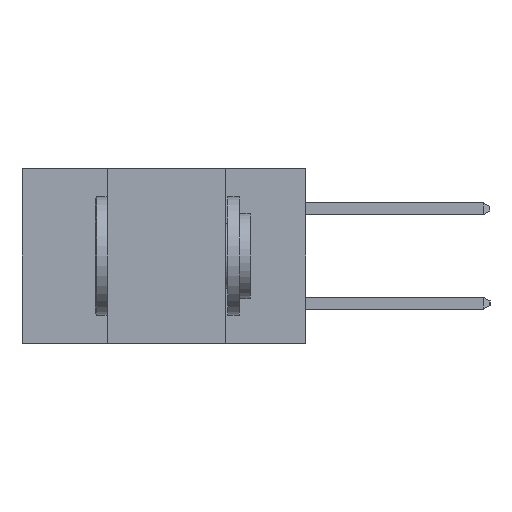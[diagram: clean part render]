
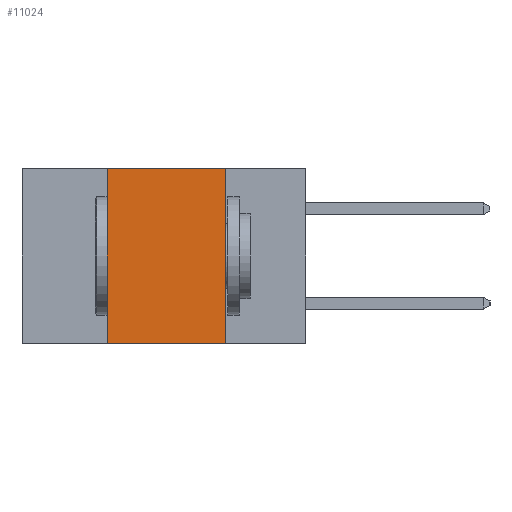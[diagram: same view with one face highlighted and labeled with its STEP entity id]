
A CAD part, left-side view. The second image highlights one B-rep face of the part: STEP entity #11024.
In plain terms, the highlighted planar face has unit normal (-1, 0, 0).
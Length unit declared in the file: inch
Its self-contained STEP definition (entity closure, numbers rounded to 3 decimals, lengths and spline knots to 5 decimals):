
#411 = CARTESIAN_POINT ( 'NONE',  ( 0., 0.6, 0. ) ) ;
#807 = VERTEX_POINT ( 'NONE', #8865 ) ;
#871 = VECTOR ( 'NONE', #3319, 39.37008 ) ;
#1193 = CARTESIAN_POINT ( 'NONE',  ( 0., 0.6, -0.37 ) ) ;
#2861 = VECTOR ( 'NONE', #19560, 39.37008 ) ;
#3172 = ORIENTED_EDGE ( 'NONE', *, *, #22668, .T. ) ;
#3319 = DIRECTION ( 'NONE',  ( 0., -1., 0. ) ) ;
#3367 = CARTESIAN_POINT ( 'NONE',  ( 0., 0.17, -0.37 ) ) ;
#3524 = LINE ( 'NONE', #15432, #2861 ) ;
#3663 = DIRECTION ( 'NONE',  ( 0., 0., -1. ) ) ;
#4638 = DIRECTION ( 'NONE',  ( 0., 0., -1. ) ) ;
#4787 = LINE ( 'NONE', #19013, #24238 ) ;
#7179 = ORIENTED_EDGE ( 'NONE', *, *, #15148, .F. ) ;
#7495 = CARTESIAN_POINT ( 'NONE',  ( 0., 0.42, -0.37 ) ) ;
#7552 = VECTOR ( 'NONE', #3663, 39.37008 ) ;
#8211 = LINE ( 'NONE', #11925, #7552 ) ;
#8865 = CARTESIAN_POINT ( 'NONE',  ( 0., 0.17, 0. ) ) ;
#10046 = AXIS2_PLACEMENT_3D ( 'NONE', #411, #17106, #4638 ) ;
#11024 = ADVANCED_FACE ( 'NONE', ( #21280 ), #15019, .F. ) ;
#11292 = VERTEX_POINT ( 'NONE', #3367 ) ;
#11925 = CARTESIAN_POINT ( 'NONE',  ( 0., 0.17, -0.37 ) ) ;
#12518 = VERTEX_POINT ( 'NONE', #25658 ) ;
#12918 = DIRECTION ( 'NONE',  ( 0., -1., 0. ) ) ;
#13520 = EDGE_LOOP ( 'NONE', ( #7179, #23000, #16839, #3172 ) ) ;
#15019 = PLANE ( 'NONE',  #10046 ) ;
#15148 = EDGE_CURVE ( 'NONE', #807, #11292, #8211, .T. ) ;
#15432 = CARTESIAN_POINT ( 'NONE',  ( 0., 0.42, -0.37 ) ) ;
#16839 = ORIENTED_EDGE ( 'NONE', *, *, #18507, .F. ) ;
#17106 = DIRECTION ( 'NONE',  ( 1., 0., 0. ) ) ;
#17209 = VERTEX_POINT ( 'NONE', #7495 ) ;
#18160 = LINE ( 'NONE', #1193, #871 ) ;
#18507 = EDGE_CURVE ( 'NONE', #17209, #12518, #3524, .T. ) ;
#18914 = EDGE_CURVE ( 'NONE', #12518, #807, #4787, .T. ) ;
#19013 = CARTESIAN_POINT ( 'NONE',  ( 0., 0.6, 0. ) ) ;
#19560 = DIRECTION ( 'NONE',  ( 0., 0., 1. ) ) ;
#21280 = FACE_OUTER_BOUND ( 'NONE', #13520, .T. ) ;
#22668 = EDGE_CURVE ( 'NONE', #17209, #11292, #18160, .T. ) ;
#23000 = ORIENTED_EDGE ( 'NONE', *, *, #18914, .F. ) ;
#24238 = VECTOR ( 'NONE', #12918, 39.37008 ) ;
#25658 = CARTESIAN_POINT ( 'NONE',  ( 0., 0.42, 0. ) ) ;
